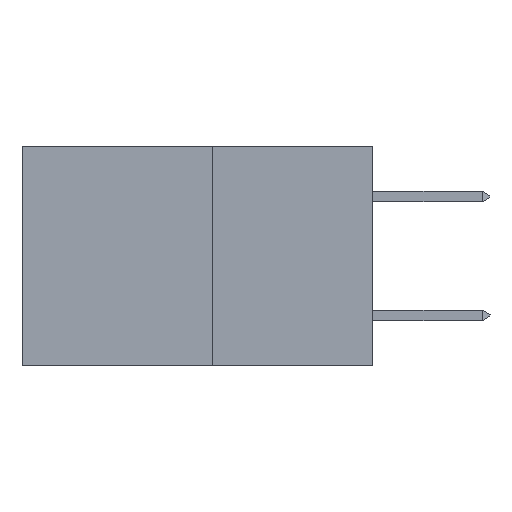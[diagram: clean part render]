
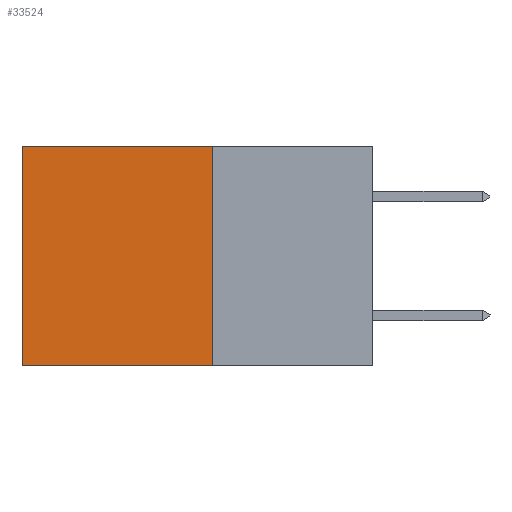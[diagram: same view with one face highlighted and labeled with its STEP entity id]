
A CAD part, left-side view. The second image highlights one B-rep face of the part: STEP entity #33524.
In plain terms, the highlighted planar face has unit normal (-1, 0, 0).
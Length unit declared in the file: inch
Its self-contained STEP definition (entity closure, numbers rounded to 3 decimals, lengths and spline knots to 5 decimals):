
#433 = LINE ( 'NONE', #8372, #1264 ) ;
#1264 = VECTOR ( 'NONE', #29325, 39.37008 ) ;
#1685 = CARTESIAN_POINT ( 'NONE',  ( 0.277, 0.27, 0. ) ) ;
#2369 = CARTESIAN_POINT ( 'NONE',  ( 0.277, 0.27, -0.37 ) ) ;
#3231 = EDGE_CURVE ( 'NONE', #19643, #32487, #26055, .T. ) ;
#4339 = DIRECTION ( 'NONE',  ( 0., 1., 0. ) ) ;
#6634 = DIRECTION ( 'NONE',  ( 0., 0., -1. ) ) ;
#7984 = LINE ( 'NONE', #1685, #14961 ) ;
#8372 = CARTESIAN_POINT ( 'NONE',  ( 0.277, 0.27, -0.37 ) ) ;
#8582 = DIRECTION ( 'NONE',  ( 0., 0., -1. ) ) ;
#9435 = EDGE_CURVE ( 'NONE', #32581, #19643, #7984, .T. ) ;
#9694 = ORIENTED_EDGE ( 'NONE', *, *, #16244, .F. ) ;
#11977 = VECTOR ( 'NONE', #8582, 39.37008 ) ;
#13268 = CARTESIAN_POINT ( 'NONE',  ( 0.277, 0.59, -0.37 ) ) ;
#14847 = FACE_OUTER_BOUND ( 'NONE', #33537, .T. ) ;
#14879 = CARTESIAN_POINT ( 'NONE',  ( 0.277, 0.59, 0. ) ) ;
#14961 = VECTOR ( 'NONE', #4339, 39.37008 ) ;
#16244 = EDGE_CURVE ( 'NONE', #32581, #28255, #28290, .T. ) ;
#16643 = ORIENTED_EDGE ( 'NONE', *, *, #9435, .T. ) ;
#18734 = DIRECTION ( 'NONE',  ( 0., 0., -1. ) ) ;
#18809 = CARTESIAN_POINT ( 'NONE',  ( 0.277, 0.59, -0.37 ) ) ;
#19643 = VERTEX_POINT ( 'NONE', #14879 ) ;
#19687 = PLANE ( 'NONE',  #30961 ) ;
#22331 = DIRECTION ( 'NONE',  ( 1., 0., 0. ) ) ;
#24702 = EDGE_CURVE ( 'NONE', #28255, #32487, #433, .T. ) ;
#26055 = LINE ( 'NONE', #18809, #32131 ) ;
#26481 = ORIENTED_EDGE ( 'NONE', *, *, #24702, .F. ) ;
#28255 = VERTEX_POINT ( 'NONE', #2369 ) ;
#28290 = LINE ( 'NONE', #32003, #11977 ) ;
#29229 = CARTESIAN_POINT ( 'NONE',  ( 0.277, 0.27, 0. ) ) ;
#29325 = DIRECTION ( 'NONE',  ( 0., 1., 0. ) ) ;
#30089 = CARTESIAN_POINT ( 'NONE',  ( 0.277, 0.27, -0.37 ) ) ;
#30961 = AXIS2_PLACEMENT_3D ( 'NONE', #30089, #22331, #6634 ) ;
#31737 = ORIENTED_EDGE ( 'NONE', *, *, #3231, .T. ) ;
#32003 = CARTESIAN_POINT ( 'NONE',  ( 0.277, 0.27, -0.37 ) ) ;
#32131 = VECTOR ( 'NONE', #18734, 39.37008 ) ;
#32487 = VERTEX_POINT ( 'NONE', #13268 ) ;
#32581 = VERTEX_POINT ( 'NONE', #29229 ) ;
#33524 = ADVANCED_FACE ( 'NONE', ( #14847 ), #19687, .F. ) ;
#33537 = EDGE_LOOP ( 'NONE', ( #31737, #26481, #9694, #16643 ) ) ;
